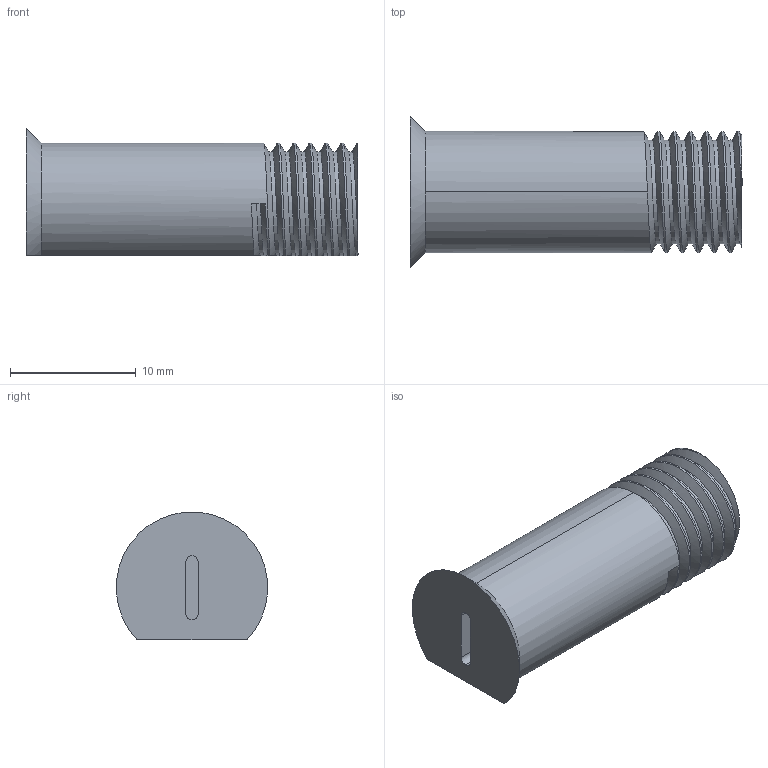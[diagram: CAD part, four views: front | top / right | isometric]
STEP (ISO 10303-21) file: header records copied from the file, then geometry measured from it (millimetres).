
FILE_DESCRIPTION (( 'STEP AP203' ), '1' );
FILE_NAME ('AF-WF-LR-PRT-006-STEP.STEP', '2020-07-21T18:16:49', ( '' ), ( '' ), 'SwSTEP 2.0', 'SolidWorks 2018', '' );
FILE_SCHEMA (( 'CONFIG_CONTROL_DESIGN' ));
Length unit declared in the file: inch
Products named in the file (1): AF-WF-LR-PRT-006-STEP
Bounding box: 26.42 x 12.04 x 10.15 mm (x, y, z)
Volume: 1796.3 mm3; surface area: 1124.6 mm2
Topology: 1 solids, 1 shells, 47 faces, 119 edges, 75 vertices
Faces by surface type: cylinder 17, bspline 16, plane 13, cone 1
Entity records: 5412 total; most frequent: CARTESIAN_POINT 4447, ORIENTED_EDGE 238, DIRECTION 121, EDGE_CURVE 119, VERTEX_POINT 75, EDGE_LOOP 48, FACE_OUTER_BOUND 47, ADVANCED_FACE 47
